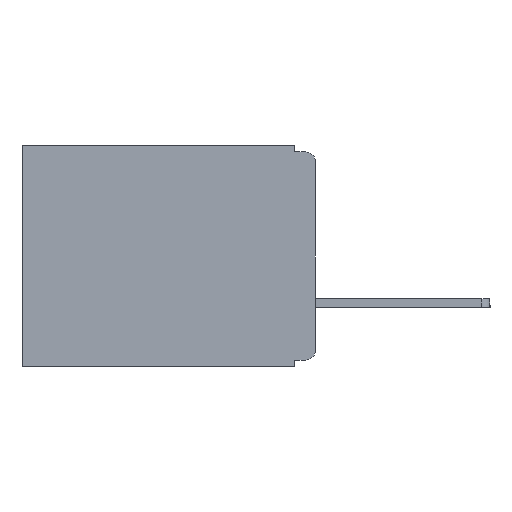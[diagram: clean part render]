
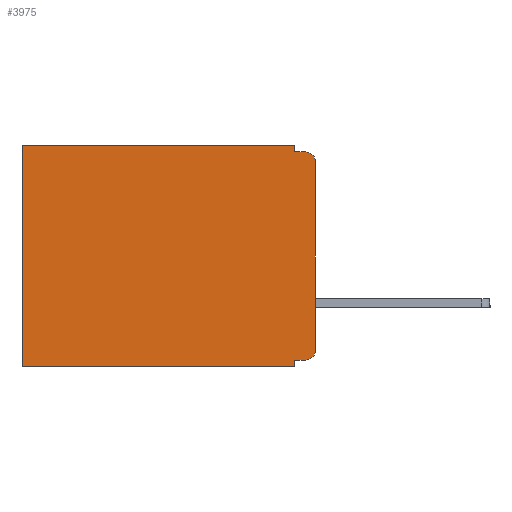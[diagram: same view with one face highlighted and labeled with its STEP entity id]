
A CAD part, left-side view. The second image highlights one B-rep face of the part: STEP entity #3975.
In plain terms, the highlighted planar face has unit normal (-1, 0, 0).
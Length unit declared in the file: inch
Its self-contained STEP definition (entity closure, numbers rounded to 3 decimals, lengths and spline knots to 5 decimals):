
#143 = EDGE_CURVE ( 'NONE', #27389, #3804, #24484, .T. ) ;
#162 = CARTESIAN_POINT ( 'NONE',  ( 0.3, 0.437, -0.33 ) ) ;
#377 = AXIS2_PLACEMENT_3D ( 'NONE', #20931, #7805, #23129 ) ;
#992 = CARTESIAN_POINT ( 'NONE',  ( 0.3, 0., -0.025 ) ) ;
#1752 = ORIENTED_EDGE ( 'NONE', *, *, #28004, .F. ) ;
#1972 = CARTESIAN_POINT ( 'NONE',  ( 0.3, 0., -0.305 ) ) ;
#2405 = DIRECTION ( 'NONE',  ( 0., 0., -1. ) ) ;
#3413 = VECTOR ( 'NONE', #15007, 39.37008 ) ;
#3559 = EDGE_CURVE ( 'NONE', #21861, #6040, #8790, .T. ) ;
#3715 = CARTESIAN_POINT ( 'NONE',  ( 0.3, 0., 0. ) ) ;
#3804 = VERTEX_POINT ( 'NONE', #23026 ) ;
#3975 = ADVANCED_FACE ( 'NONE', ( #24856 ), #25380, .F. ) ;
#4615 = DIRECTION ( 'NONE',  ( -1., 0., 0. ) ) ;
#5210 = VERTEX_POINT ( 'NONE', #7448 ) ;
#5891 = CARTESIAN_POINT ( 'NONE',  ( 0.3, 0.031, 0. ) ) ;
#6040 = VERTEX_POINT ( 'NONE', #1972 ) ;
#7448 = CARTESIAN_POINT ( 'NONE',  ( 0.3, 0.015, -0.01 ) ) ;
#7805 = DIRECTION ( 'NONE',  ( -1., 0., 0. ) ) ;
#7824 = EDGE_CURVE ( 'NONE', #19333, #15741, #9878, .T. ) ;
#8525 = DIRECTION ( 'NONE',  ( 0., -1., 0. ) ) ;
#8554 = CARTESIAN_POINT ( 'NONE',  ( 0.3, 0., -0.01 ) ) ;
#8630 = ORIENTED_EDGE ( 'NONE', *, *, #143, .F. ) ;
#8790 = LINE ( 'NONE', #21285, #19090 ) ;
#9878 = LINE ( 'NONE', #16624, #26660 ) ;
#10435 = CARTESIAN_POINT ( 'NONE',  ( 0.3, 0.031, -0.32 ) ) ;
#11009 = ORIENTED_EDGE ( 'NONE', *, *, #18189, .T. ) ;
#12342 = CARTESIAN_POINT ( 'NONE',  ( 0.3, 0.437, -0.33 ) ) ;
#12453 = EDGE_CURVE ( 'NONE', #15741, #5210, #26334, .T. ) ;
#13220 = VERTEX_POINT ( 'NONE', #17572 ) ;
#13421 = LINE ( 'NONE', #162, #19275 ) ;
#14168 = EDGE_LOOP ( 'NONE', ( #22254, #23608, #24208, #26179, #26874, #27208, #1752, #8630, #27432, #11009 ) ) ;
#14442 = EDGE_CURVE ( 'NONE', #21861, #5210, #18046, .T. ) ;
#14995 = LINE ( 'NONE', #28076, #3413 ) ;
#15007 = DIRECTION ( 'NONE',  ( 0., 1., 0. ) ) ;
#15272 = CIRCLE ( 'NONE', #377, 0.015 ) ;
#15741 = VERTEX_POINT ( 'NONE', #24336 ) ;
#16009 = CARTESIAN_POINT ( 'NONE',  ( 0.3, 0.031, -0.33 ) ) ;
#16265 = DIRECTION ( 'NONE',  ( 0., 0., -1. ) ) ;
#16478 = EDGE_CURVE ( 'NONE', #19333, #13220, #19498, .T. ) ;
#16624 = CARTESIAN_POINT ( 'NONE',  ( 0.3, 0.031, 0. ) ) ;
#17535 = LINE ( 'NONE', #20936, #21984 ) ;
#17572 = CARTESIAN_POINT ( 'NONE',  ( 0.3, 0.437, 0. ) ) ;
#17694 = CARTESIAN_POINT ( 'NONE',  ( 0.3, 0.015, -0.025 ) ) ;
#17725 = AXIS2_PLACEMENT_3D ( 'NONE', #17694, #4615, #19912 ) ;
#17871 = DIRECTION ( 'NONE',  ( 0., 0., -1. ) ) ;
#18046 = CIRCLE ( 'NONE', #17725, 0.015 ) ;
#18119 = CARTESIAN_POINT ( 'NONE',  ( 0.3, 0., -0.33 ) ) ;
#18189 = EDGE_CURVE ( 'NONE', #26555, #6040, #15272, .T. ) ;
#18619 = DIRECTION ( 'NONE',  ( 0., 0., -1. ) ) ;
#18874 = DIRECTION ( 'NONE',  ( 0., 0., -1. ) ) ;
#19002 = DIRECTION ( 'NONE',  ( 0., 1., 0. ) ) ;
#19090 = VECTOR ( 'NONE', #18874, 39.37008 ) ;
#19275 = VECTOR ( 'NONE', #2405, 39.37008 ) ;
#19333 = VERTEX_POINT ( 'NONE', #5891 ) ;
#19498 = LINE ( 'NONE', #3715, #24608 ) ;
#19912 = DIRECTION ( 'NONE',  ( 0., 0., -1. ) ) ;
#20549 = VECTOR ( 'NONE', #8525, 39.37008 ) ;
#20702 = EDGE_CURVE ( 'NONE', #13220, #27879, #13421, .T. ) ;
#20931 = CARTESIAN_POINT ( 'NONE',  ( 0.3, 0.015, -0.305 ) ) ;
#20936 = CARTESIAN_POINT ( 'NONE',  ( 0.3, 0., -0.32 ) ) ;
#21006 = EDGE_CURVE ( 'NONE', #26555, #27389, #17535, .T. ) ;
#21285 = CARTESIAN_POINT ( 'NONE',  ( 0.3, 0., -0.33 ) ) ;
#21861 = VERTEX_POINT ( 'NONE', #992 ) ;
#21984 = VECTOR ( 'NONE', #23135, 39.37008 ) ;
#22254 = ORIENTED_EDGE ( 'NONE', *, *, #3559, .F. ) ;
#23026 = CARTESIAN_POINT ( 'NONE',  ( 0.3, 0.031, -0.33 ) ) ;
#23129 = DIRECTION ( 'NONE',  ( 0., 0., -1. ) ) ;
#23135 = DIRECTION ( 'NONE',  ( 0., 1., 0. ) ) ;
#23608 = ORIENTED_EDGE ( 'NONE', *, *, #14442, .T. ) ;
#23803 = VECTOR ( 'NONE', #17871, 39.37008 ) ;
#24208 = ORIENTED_EDGE ( 'NONE', *, *, #12453, .F. ) ;
#24336 = CARTESIAN_POINT ( 'NONE',  ( 0.3, 0.031, -0.01 ) ) ;
#24484 = LINE ( 'NONE', #16009, #23803 ) ;
#24608 = VECTOR ( 'NONE', #19002, 39.37008 ) ;
#24640 = DIRECTION ( 'NONE',  ( 1., 0., 0. ) ) ;
#24856 = FACE_OUTER_BOUND ( 'NONE', #14168, .T. ) ;
#25210 = AXIS2_PLACEMENT_3D ( 'NONE', #18119, #24640, #18619 ) ;
#25380 = PLANE ( 'NONE',  #25210 ) ;
#26179 = ORIENTED_EDGE ( 'NONE', *, *, #7824, .F. ) ;
#26334 = LINE ( 'NONE', #8554, #20549 ) ;
#26542 = CARTESIAN_POINT ( 'NONE',  ( 0.3, 0.015, -0.32 ) ) ;
#26555 = VERTEX_POINT ( 'NONE', #26542 ) ;
#26660 = VECTOR ( 'NONE', #16265, 39.37008 ) ;
#26874 = ORIENTED_EDGE ( 'NONE', *, *, #16478, .T. ) ;
#27208 = ORIENTED_EDGE ( 'NONE', *, *, #20702, .T. ) ;
#27389 = VERTEX_POINT ( 'NONE', #10435 ) ;
#27432 = ORIENTED_EDGE ( 'NONE', *, *, #21006, .F. ) ;
#27879 = VERTEX_POINT ( 'NONE', #12342 ) ;
#28004 = EDGE_CURVE ( 'NONE', #3804, #27879, #14995, .T. ) ;
#28076 = CARTESIAN_POINT ( 'NONE',  ( 0.3, 0., -0.33 ) ) ;
